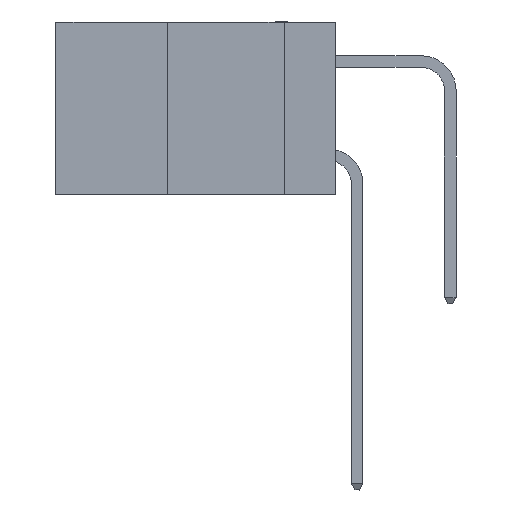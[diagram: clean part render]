
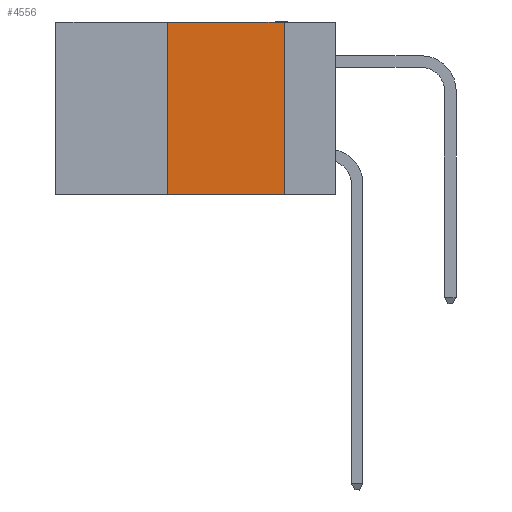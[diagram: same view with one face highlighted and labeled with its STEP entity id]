
A CAD part, left-side view. The second image highlights one B-rep face of the part: STEP entity #4556.
In plain terms, the highlighted planar face has unit normal (-1, 0, 0).
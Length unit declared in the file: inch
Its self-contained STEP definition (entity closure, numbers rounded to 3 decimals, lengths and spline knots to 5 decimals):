
#523 = EDGE_CURVE ( 'NONE', #2185, #18490, #27010, .T. ) ;
#2185 = VERTEX_POINT ( 'NONE', #29668 ) ;
#4556 = ADVANCED_FACE ( 'NONE', ( #8997 ), #34090, .F. ) ;
#4833 = VERTEX_POINT ( 'NONE', #19459 ) ;
#4840 = AXIS2_PLACEMENT_3D ( 'NONE', #27566, #24428, #17720 ) ;
#8433 = VERTEX_POINT ( 'NONE', #42015 ) ;
#8635 = DIRECTION ( 'NONE',  ( 0., 0., 1. ) ) ;
#8997 = FACE_OUTER_BOUND ( 'NONE', #10572, .T. ) ;
#9266 = EDGE_CURVE ( 'NONE', #4833, #2185, #35555, .T. ) ;
#9768 = DIRECTION ( 'NONE',  ( 0., -1., 0. ) ) ;
#10572 = EDGE_LOOP ( 'NONE', ( #10818, #16882, #44195, #42104 ) ) ;
#10818 = ORIENTED_EDGE ( 'NONE', *, *, #15092, .F. ) ;
#11585 = CARTESIAN_POINT ( 'NONE',  ( 0., 0.11, 0. ) ) ;
#12231 = CARTESIAN_POINT ( 'NONE',  ( 0., 0.36, 0. ) ) ;
#12402 = DIRECTION ( 'NONE',  ( 0., -1., 0. ) ) ;
#15092 = EDGE_CURVE ( 'NONE', #18490, #8433, #38513, .T. ) ;
#15775 = CARTESIAN_POINT ( 'NONE',  ( 0., 0.6, -0.37 ) ) ;
#16882 = ORIENTED_EDGE ( 'NONE', *, *, #523, .F. ) ;
#17164 = CARTESIAN_POINT ( 'NONE',  ( 0., 0.6, 0. ) ) ;
#17632 = CARTESIAN_POINT ( 'NONE',  ( 0., 0.11, 0. ) ) ;
#17720 = DIRECTION ( 'NONE',  ( 0., 0., -1. ) ) ;
#18490 = VERTEX_POINT ( 'NONE', #17632 ) ;
#18670 = VECTOR ( 'NONE', #12402, 39.37008 ) ;
#19459 = CARTESIAN_POINT ( 'NONE',  ( 0., 0.36, -0.37 ) ) ;
#21391 = VECTOR ( 'NONE', #9768, 39.37008 ) ;
#24428 = DIRECTION ( 'NONE',  ( 1., 0., 0. ) ) ;
#26712 = VECTOR ( 'NONE', #28616, 39.37008 ) ;
#26714 = LINE ( 'NONE', #15775, #18670 ) ;
#26883 = VECTOR ( 'NONE', #8635, 39.37008 ) ;
#27010 = LINE ( 'NONE', #17164, #21391 ) ;
#27566 = CARTESIAN_POINT ( 'NONE',  ( 0., 0.6, 0. ) ) ;
#28616 = DIRECTION ( 'NONE',  ( 0., 0., -1. ) ) ;
#29668 = CARTESIAN_POINT ( 'NONE',  ( 0., 0.36, 0. ) ) ;
#30246 = EDGE_CURVE ( 'NONE', #4833, #8433, #26714, .T. ) ;
#34090 = PLANE ( 'NONE',  #4840 ) ;
#35555 = LINE ( 'NONE', #12231, #26883 ) ;
#38513 = LINE ( 'NONE', #11585, #26712 ) ;
#42015 = CARTESIAN_POINT ( 'NONE',  ( 0., 0.11, -0.37 ) ) ;
#42104 = ORIENTED_EDGE ( 'NONE', *, *, #30246, .T. ) ;
#44195 = ORIENTED_EDGE ( 'NONE', *, *, #9266, .F. ) ;
